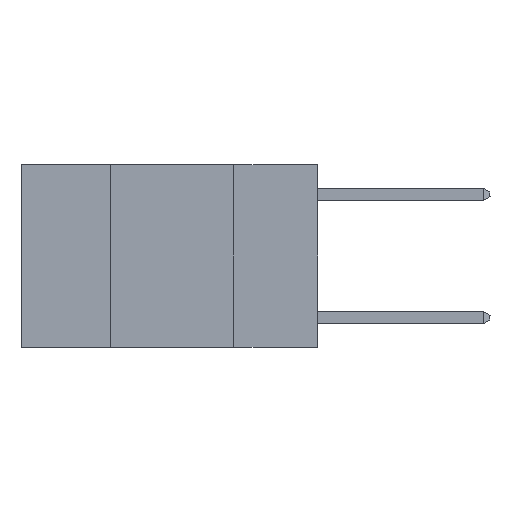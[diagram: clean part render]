
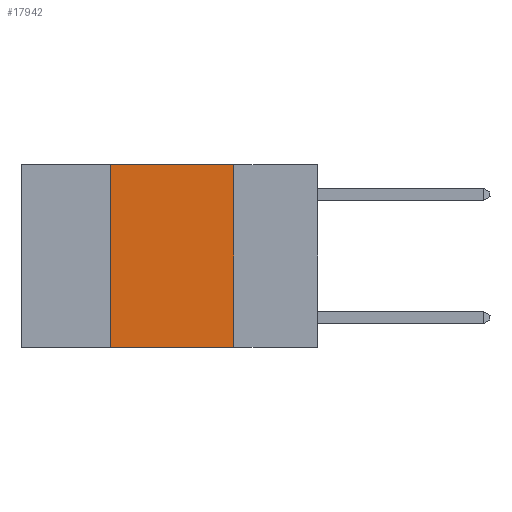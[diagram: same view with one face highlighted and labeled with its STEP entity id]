
A CAD part, left-side view. The second image highlights one B-rep face of the part: STEP entity #17942.
In plain terms, the highlighted planar face has unit normal (-1, 0, 0).
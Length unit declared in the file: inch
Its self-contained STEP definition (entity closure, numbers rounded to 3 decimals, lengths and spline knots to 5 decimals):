
#1027 = VECTOR ( 'NONE', #13637, 39.37008 ) ;
#1929 = CARTESIAN_POINT ( 'NONE',  ( 0., 0.42, 0. ) ) ;
#2915 = CARTESIAN_POINT ( 'NONE',  ( 0., 0.17, 0. ) ) ;
#3179 = DIRECTION ( 'NONE',  ( 1., 0., 0. ) ) ;
#3268 = CARTESIAN_POINT ( 'NONE',  ( 0., 0.42, 0. ) ) ;
#3302 = CARTESIAN_POINT ( 'NONE',  ( 0., 0.42, -0.37 ) ) ;
#3783 = EDGE_CURVE ( 'NONE', #20680, #8556, #14699, .T. ) ;
#3849 = CARTESIAN_POINT ( 'NONE',  ( 0., 0.6, 0. ) ) ;
#5420 = EDGE_CURVE ( 'NONE', #19873, #8556, #21586, .T. ) ;
#5742 = EDGE_CURVE ( 'NONE', #20680, #6103, #6858, .T. ) ;
#6103 = VERTEX_POINT ( 'NONE', #3268 ) ;
#6858 = LINE ( 'NONE', #1929, #16462 ) ;
#8556 = VERTEX_POINT ( 'NONE', #14934 ) ;
#8902 = EDGE_CURVE ( 'NONE', #6103, #19873, #13997, .T. ) ;
#10004 = PLANE ( 'NONE',  #17306 ) ;
#12755 = VECTOR ( 'NONE', #18196, 39.37008 ) ;
#13070 = CARTESIAN_POINT ( 'NONE',  ( 0., 0.17, 0. ) ) ;
#13382 = ORIENTED_EDGE ( 'NONE', *, *, #5420, .F. ) ;
#13448 = ORIENTED_EDGE ( 'NONE', *, *, #8902, .F. ) ;
#13580 = EDGE_LOOP ( 'NONE', ( #13382, #13448, #14123, #14134 ) ) ;
#13637 = DIRECTION ( 'NONE',  ( 0., -1., 0. ) ) ;
#13997 = LINE ( 'NONE', #3849, #17940 ) ;
#14123 = ORIENTED_EDGE ( 'NONE', *, *, #5742, .F. ) ;
#14134 = ORIENTED_EDGE ( 'NONE', *, *, #3783, .T. ) ;
#14699 = LINE ( 'NONE', #20247, #1027 ) ;
#14934 = CARTESIAN_POINT ( 'NONE',  ( 0., 0.17, -0.37 ) ) ;
#15138 = DIRECTION ( 'NONE',  ( 0., 0., -1. ) ) ;
#16462 = VECTOR ( 'NONE', #17319, 39.37008 ) ;
#17306 = AXIS2_PLACEMENT_3D ( 'NONE', #20081, #3179, #15138 ) ;
#17319 = DIRECTION ( 'NONE',  ( 0., 0., 1. ) ) ;
#17910 = FACE_OUTER_BOUND ( 'NONE', #13580, .T. ) ;
#17940 = VECTOR ( 'NONE', #19161, 39.37008 ) ;
#17942 = ADVANCED_FACE ( 'NONE', ( #17910 ), #10004, .F. ) ;
#18196 = DIRECTION ( 'NONE',  ( 0., 0., -1. ) ) ;
#19161 = DIRECTION ( 'NONE',  ( 0., -1., 0. ) ) ;
#19873 = VERTEX_POINT ( 'NONE', #13070 ) ;
#20081 = CARTESIAN_POINT ( 'NONE',  ( 0., 0.6, 0. ) ) ;
#20247 = CARTESIAN_POINT ( 'NONE',  ( 0., 0.6, -0.37 ) ) ;
#20680 = VERTEX_POINT ( 'NONE', #3302 ) ;
#21586 = LINE ( 'NONE', #2915, #12755 ) ;
